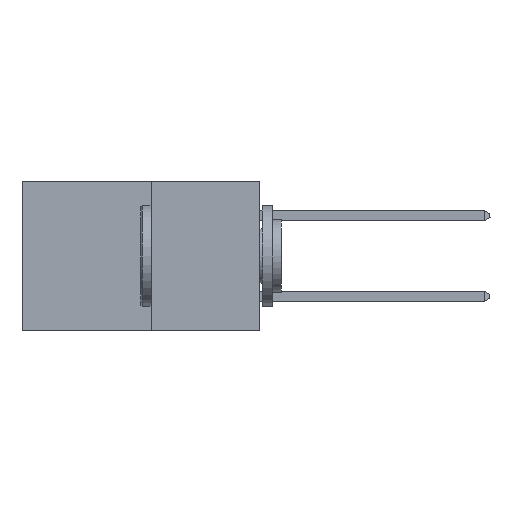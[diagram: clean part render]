
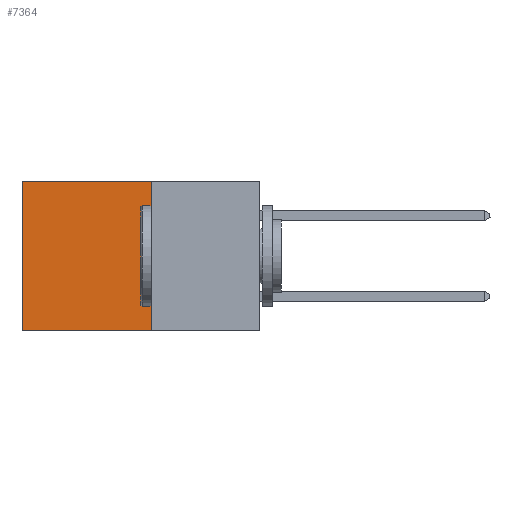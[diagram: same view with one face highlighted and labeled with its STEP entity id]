
A CAD part, left-side view. The second image highlights one B-rep face of the part: STEP entity #7364.
In plain terms, the highlighted planar face has unit normal (-1, 0, 0).
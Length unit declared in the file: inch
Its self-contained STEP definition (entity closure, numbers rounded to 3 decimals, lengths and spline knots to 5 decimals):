
#508 = EDGE_LOOP ( 'NONE', ( #8580, #10163, #23224, #25762 ) ) ;
#1182 = CARTESIAN_POINT ( 'NONE',  ( 0.277, 0.27, -0.37 ) ) ;
#1610 = CARTESIAN_POINT ( 'NONE',  ( 0.277, 0.27, -0.37 ) ) ;
#2759 = LINE ( 'NONE', #7528, #19922 ) ;
#3907 = DIRECTION ( 'NONE',  ( 0., 1., 0. ) ) ;
#4079 = EDGE_CURVE ( 'NONE', #28470, #9069, #20197, .T. ) ;
#7364 = ADVANCED_FACE ( 'NONE', ( #20303 ), #25828, .F. ) ;
#7528 = CARTESIAN_POINT ( 'NONE',  ( 0.277, 0.59, -0.37 ) ) ;
#7818 = CARTESIAN_POINT ( 'NONE',  ( 0.277, 0.59, -0.37 ) ) ;
#8047 = EDGE_CURVE ( 'NONE', #9069, #26766, #2759, .T. ) ;
#8083 = DIRECTION ( 'NONE',  ( 0., 0., -1. ) ) ;
#8229 = VECTOR ( 'NONE', #23472, 39.37008 ) ;
#8272 = VECTOR ( 'NONE', #18946, 39.37008 ) ;
#8580 = ORIENTED_EDGE ( 'NONE', *, *, #8047, .T. ) ;
#9069 = VERTEX_POINT ( 'NONE', #21054 ) ;
#10163 = ORIENTED_EDGE ( 'NONE', *, *, #23685, .F. ) ;
#10880 = CARTESIAN_POINT ( 'NONE',  ( 0.277, 0.27, 0. ) ) ;
#11328 = CARTESIAN_POINT ( 'NONE',  ( 0.277, 0.27, -0.37 ) ) ;
#11679 = LINE ( 'NONE', #1610, #16966 ) ;
#13341 = VERTEX_POINT ( 'NONE', #11328 ) ;
#13678 = EDGE_CURVE ( 'NONE', #28470, #13341, #14172, .T. ) ;
#14172 = LINE ( 'NONE', #1182, #8229 ) ;
#16966 = VECTOR ( 'NONE', #3907, 39.37008 ) ;
#18946 = DIRECTION ( 'NONE',  ( 0., 1., 0. ) ) ;
#19526 = CARTESIAN_POINT ( 'NONE',  ( 0.277, 0.27, 0. ) ) ;
#19922 = VECTOR ( 'NONE', #8083, 39.37008 ) ;
#20197 = LINE ( 'NONE', #19526, #8272 ) ;
#20303 = FACE_OUTER_BOUND ( 'NONE', #508, .T. ) ;
#21054 = CARTESIAN_POINT ( 'NONE',  ( 0.277, 0.59, 0. ) ) ;
#23224 = ORIENTED_EDGE ( 'NONE', *, *, #13678, .F. ) ;
#23472 = DIRECTION ( 'NONE',  ( 0., 0., -1. ) ) ;
#23685 = EDGE_CURVE ( 'NONE', #13341, #26766, #11679, .T. ) ;
#23832 = AXIS2_PLACEMENT_3D ( 'NONE', #25747, #25661, #25656 ) ;
#25656 = DIRECTION ( 'NONE',  ( 0., 0., -1. ) ) ;
#25661 = DIRECTION ( 'NONE',  ( 1., 0., 0. ) ) ;
#25747 = CARTESIAN_POINT ( 'NONE',  ( 0.277, 0.27, -0.37 ) ) ;
#25762 = ORIENTED_EDGE ( 'NONE', *, *, #4079, .T. ) ;
#25828 = PLANE ( 'NONE',  #23832 ) ;
#26766 = VERTEX_POINT ( 'NONE', #7818 ) ;
#28470 = VERTEX_POINT ( 'NONE', #10880 ) ;
